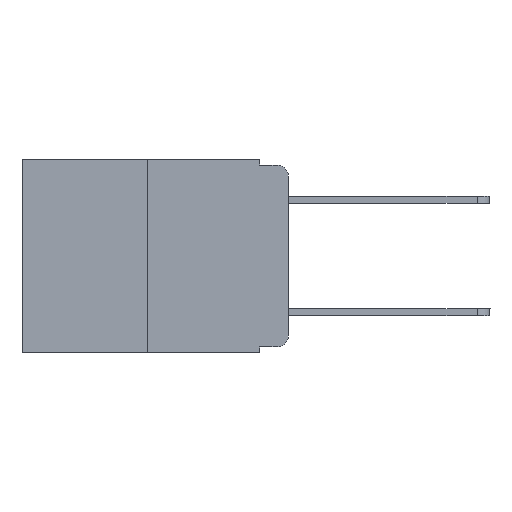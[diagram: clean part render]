
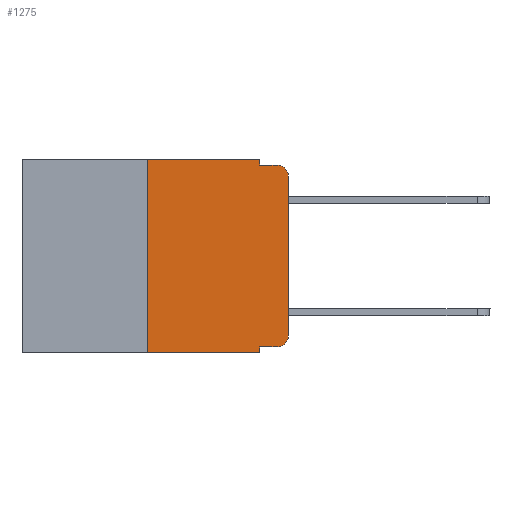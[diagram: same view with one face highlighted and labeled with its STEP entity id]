
A CAD part, left-side view. The second image highlights one B-rep face of the part: STEP entity #1275.
In plain terms, the highlighted planar face has unit normal (-1, 0, 0).
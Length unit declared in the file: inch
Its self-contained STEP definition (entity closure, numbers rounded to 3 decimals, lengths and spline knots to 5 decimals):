
#47 = LINE ( 'NONE', #13343, #12130 ) ;
#251 = VERTEX_POINT ( 'NONE', #11484 ) ;
#413 = CARTESIAN_POINT ( 'NONE',  ( 0., 0.051, -0.333 ) ) ;
#502 = EDGE_CURVE ( 'NONE', #251, #1077, #2560, .T. ) ;
#1077 = VERTEX_POINT ( 'NONE', #2606 ) ;
#1103 = LINE ( 'NONE', #12357, #5544 ) ;
#1275 = ADVANCED_FACE ( 'NONE', ( #4447 ), #8364, .F. ) ;
#1292 = EDGE_CURVE ( 'NONE', #8037, #3394, #11338, .T. ) ;
#1387 = VECTOR ( 'NONE', #2832, 39.37008 ) ;
#1521 = EDGE_CURVE ( 'NONE', #11375, #14625, #1546, .T. ) ;
#1546 = LINE ( 'NONE', #13151, #14795 ) ;
#2372 = VERTEX_POINT ( 'NONE', #10224 ) ;
#2560 = LINE ( 'NONE', #413, #1387 ) ;
#2606 = CARTESIAN_POINT ( 'NONE',  ( 0., 0.02, -0.333 ) ) ;
#2832 = DIRECTION ( 'NONE',  ( 0., -1., 0. ) ) ;
#3303 = VECTOR ( 'NONE', #10831, 39.37008 ) ;
#3394 = VERTEX_POINT ( 'NONE', #3467 ) ;
#3449 = EDGE_CURVE ( 'NONE', #2372, #6014, #13789, .T. ) ;
#3467 = CARTESIAN_POINT ( 'NONE',  ( 0., 0.02, -0.01 ) ) ;
#3550 = ORIENTED_EDGE ( 'NONE', *, *, #6120, .T. ) ;
#3613 = ORIENTED_EDGE ( 'NONE', *, *, #12618, .F. ) ;
#3753 = DIRECTION ( 'NONE',  ( 0., 0., 1. ) ) ;
#3830 = CARTESIAN_POINT ( 'NONE',  ( 0., 0.051, 0. ) ) ;
#3934 = AXIS2_PLACEMENT_3D ( 'NONE', #13941, #8850, #5343 ) ;
#4188 = EDGE_LOOP ( 'NONE', ( #10869, #3550, #13783, #15830, #4907, #6106, #14518, #3613, #14510, #10250 ) ) ;
#4447 = FACE_OUTER_BOUND ( 'NONE', #4188, .T. ) ;
#4907 = ORIENTED_EDGE ( 'NONE', *, *, #1521, .F. ) ;
#5038 = CARTESIAN_POINT ( 'NONE',  ( 0., 0.051, 0. ) ) ;
#5343 = DIRECTION ( 'NONE',  ( 0., 0., -1. ) ) ;
#5383 = DIRECTION ( 'NONE',  ( 0., 0., -1. ) ) ;
#5544 = VECTOR ( 'NONE', #11208, 39.37008 ) ;
#5554 = CARTESIAN_POINT ( 'NONE',  ( 0., 0., 0. ) ) ;
#5621 = CIRCLE ( 'NONE', #3934, 0.02 ) ;
#5831 = DIRECTION ( 'NONE',  ( 0., -1., 0. ) ) ;
#5863 = CARTESIAN_POINT ( 'NONE',  ( 0., 0.051, -0.01 ) ) ;
#5982 = DIRECTION ( 'NONE',  ( 1., 0., 0. ) ) ;
#6014 = VERTEX_POINT ( 'NONE', #13720 ) ;
#6106 = ORIENTED_EDGE ( 'NONE', *, *, #7081, .F. ) ;
#6120 = EDGE_CURVE ( 'NONE', #14080, #3394, #11187, .T. ) ;
#6379 = LINE ( 'NONE', #5554, #10934 ) ;
#7081 = EDGE_CURVE ( 'NONE', #2372, #11375, #47, .T. ) ;
#7170 = CARTESIAN_POINT ( 'NONE',  ( 0., 0., -0.313 ) ) ;
#7283 = CARTESIAN_POINT ( 'NONE',  ( 0., 0.473, 0. ) ) ;
#8037 = VERTEX_POINT ( 'NONE', #5863 ) ;
#8093 = VECTOR ( 'NONE', #9848, 39.37008 ) ;
#8315 = DIRECTION ( 'NONE',  ( 0., 0., -1. ) ) ;
#8364 = PLANE ( 'NONE',  #13660 ) ;
#8850 = DIRECTION ( 'NONE',  ( -1., 0., 0. ) ) ;
#9430 = CARTESIAN_POINT ( 'NONE',  ( 0., 0.473, -0.343 ) ) ;
#9607 = CARTESIAN_POINT ( 'NONE',  ( 0., 0.051, -0.01 ) ) ;
#9848 = DIRECTION ( 'NONE',  ( 0., 0., -1. ) ) ;
#10224 = CARTESIAN_POINT ( 'NONE',  ( 0., 0.25, -0.343 ) ) ;
#10250 = ORIENTED_EDGE ( 'NONE', *, *, #12723, .T. ) ;
#10257 = CARTESIAN_POINT ( 'NONE',  ( 0., 0.02, -0.03 ) ) ;
#10305 = DIRECTION ( 'NONE',  ( -1., 0., 0. ) ) ;
#10831 = DIRECTION ( 'NONE',  ( 0., -1., 0. ) ) ;
#10869 = ORIENTED_EDGE ( 'NONE', *, *, #12916, .T. ) ;
#10934 = VECTOR ( 'NONE', #15342, 39.37008 ) ;
#10936 = CARTESIAN_POINT ( 'NONE',  ( 0., 0.25, 0. ) ) ;
#10954 = LINE ( 'NONE', #3830, #8093 ) ;
#11187 = CIRCLE ( 'NONE', #12599, 0.02 ) ;
#11208 = DIRECTION ( 'NONE',  ( 0., 0., -1. ) ) ;
#11338 = LINE ( 'NONE', #9607, #3303 ) ;
#11375 = VERTEX_POINT ( 'NONE', #10936 ) ;
#11484 = CARTESIAN_POINT ( 'NONE',  ( 0., 0.051, -0.333 ) ) ;
#12130 = VECTOR ( 'NONE', #3753, 39.37008 ) ;
#12357 = CARTESIAN_POINT ( 'NONE',  ( 0., 0.051, 0. ) ) ;
#12599 = AXIS2_PLACEMENT_3D ( 'NONE', #10257, #10305, #5383 ) ;
#12618 = EDGE_CURVE ( 'NONE', #251, #6014, #10954, .T. ) ;
#12723 = EDGE_CURVE ( 'NONE', #1077, #12933, #5621, .T. ) ;
#12916 = EDGE_CURVE ( 'NONE', #12933, #14080, #6379, .T. ) ;
#12933 = VERTEX_POINT ( 'NONE', #7170 ) ;
#13102 = CARTESIAN_POINT ( 'NONE',  ( 0., 0., -0.03 ) ) ;
#13151 = CARTESIAN_POINT ( 'NONE',  ( 0., 0.473, 0. ) ) ;
#13343 = CARTESIAN_POINT ( 'NONE',  ( 0., 0.25, 0. ) ) ;
#13400 = VECTOR ( 'NONE', #14262, 39.37008 ) ;
#13660 = AXIS2_PLACEMENT_3D ( 'NONE', #7283, #5982, #8315 ) ;
#13720 = CARTESIAN_POINT ( 'NONE',  ( 0., 0.051, -0.343 ) ) ;
#13783 = ORIENTED_EDGE ( 'NONE', *, *, #1292, .F. ) ;
#13789 = LINE ( 'NONE', #9430, #13400 ) ;
#13941 = CARTESIAN_POINT ( 'NONE',  ( 0., 0.02, -0.313 ) ) ;
#14080 = VERTEX_POINT ( 'NONE', #13102 ) ;
#14262 = DIRECTION ( 'NONE',  ( 0., -1., 0. ) ) ;
#14510 = ORIENTED_EDGE ( 'NONE', *, *, #502, .T. ) ;
#14518 = ORIENTED_EDGE ( 'NONE', *, *, #3449, .T. ) ;
#14625 = VERTEX_POINT ( 'NONE', #5038 ) ;
#14795 = VECTOR ( 'NONE', #5831, 39.37008 ) ;
#15215 = EDGE_CURVE ( 'NONE', #14625, #8037, #1103, .T. ) ;
#15342 = DIRECTION ( 'NONE',  ( 0., 0., 1. ) ) ;
#15830 = ORIENTED_EDGE ( 'NONE', *, *, #15215, .F. ) ;
